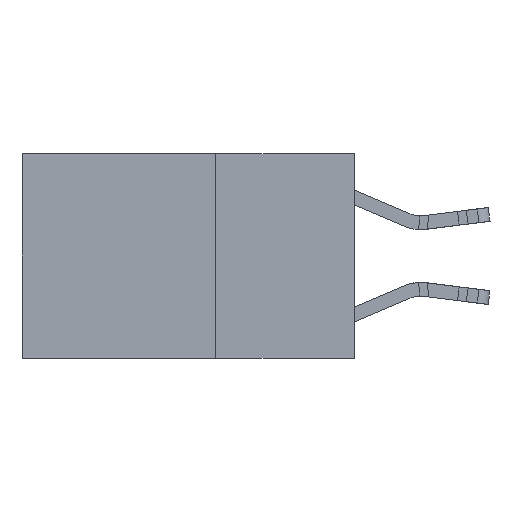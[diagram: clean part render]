
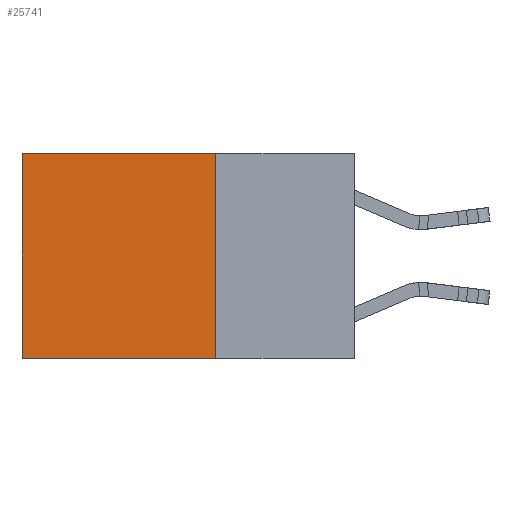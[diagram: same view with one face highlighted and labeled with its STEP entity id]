
A CAD part, left-side view. The second image highlights one B-rep face of the part: STEP entity #25741.
In plain terms, the highlighted planar face has unit normal (-1, 0, 0).
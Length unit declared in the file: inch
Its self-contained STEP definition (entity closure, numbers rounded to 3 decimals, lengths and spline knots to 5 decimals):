
#774 = VECTOR ( 'NONE', #12331, 39.37008 ) ;
#1346 = VERTEX_POINT ( 'NONE', #7805 ) ;
#3901 = LINE ( 'NONE', #20102, #15450 ) ;
#4972 = LINE ( 'NONE', #28841, #12006 ) ;
#5324 = DIRECTION ( 'NONE',  ( 0., 0., -1. ) ) ;
#5791 = ORIENTED_EDGE ( 'NONE', *, *, #26344, .F. ) ;
#7805 = CARTESIAN_POINT ( 'NONE',  ( 0.2625, 0.25, -0.37 ) ) ;
#8162 = VERTEX_POINT ( 'NONE', #11257 ) ;
#8326 = EDGE_CURVE ( 'NONE', #1346, #24345, #26204, .T. ) ;
#10765 = LINE ( 'NONE', #12614, #16415 ) ;
#11257 = CARTESIAN_POINT ( 'NONE',  ( 0.2625, 0.6, 0. ) ) ;
#12006 = VECTOR ( 'NONE', #23373, 39.37008 ) ;
#12331 = DIRECTION ( 'NONE',  ( 0., 1., 0. ) ) ;
#12614 = CARTESIAN_POINT ( 'NONE',  ( 0.2625, 0.25, 0. ) ) ;
#12901 = EDGE_LOOP ( 'NONE', ( #26995, #19051, #5791, #21769 ) ) ;
#13776 = EDGE_CURVE ( 'NONE', #8162, #24345, #4972, .T. ) ;
#14647 = CARTESIAN_POINT ( 'NONE',  ( 0.2625, 0.25, -0.37 ) ) ;
#14826 = DIRECTION ( 'NONE',  ( 1., 0., 0. ) ) ;
#15252 = DIRECTION ( 'NONE',  ( 0., 0., -1. ) ) ;
#15409 = DIRECTION ( 'NONE',  ( 0., 1., 0. ) ) ;
#15450 = VECTOR ( 'NONE', #15409, 39.37008 ) ;
#16415 = VECTOR ( 'NONE', #15252, 39.37008 ) ;
#16723 = FACE_OUTER_BOUND ( 'NONE', #12901, .T. ) ;
#17177 = PLANE ( 'NONE',  #27354 ) ;
#19051 = ORIENTED_EDGE ( 'NONE', *, *, #8326, .F. ) ;
#20066 = VERTEX_POINT ( 'NONE', #28333 ) ;
#20102 = CARTESIAN_POINT ( 'NONE',  ( 0.2625, 0.25, 0. ) ) ;
#21769 = ORIENTED_EDGE ( 'NONE', *, *, #27733, .T. ) ;
#21981 = CARTESIAN_POINT ( 'NONE',  ( 0.2625, 0.6, -0.37 ) ) ;
#23373 = DIRECTION ( 'NONE',  ( 0., 0., -1. ) ) ;
#24345 = VERTEX_POINT ( 'NONE', #21981 ) ;
#25741 = ADVANCED_FACE ( 'NONE', ( #16723 ), #17177, .F. ) ;
#26204 = LINE ( 'NONE', #14647, #774 ) ;
#26344 = EDGE_CURVE ( 'NONE', #20066, #1346, #10765, .T. ) ;
#26845 = CARTESIAN_POINT ( 'NONE',  ( 0.2625, 0.25, 0. ) ) ;
#26995 = ORIENTED_EDGE ( 'NONE', *, *, #13776, .T. ) ;
#27354 = AXIS2_PLACEMENT_3D ( 'NONE', #26845, #14826, #5324 ) ;
#27733 = EDGE_CURVE ( 'NONE', #20066, #8162, #3901, .T. ) ;
#28333 = CARTESIAN_POINT ( 'NONE',  ( 0.2625, 0.25, 0. ) ) ;
#28841 = CARTESIAN_POINT ( 'NONE',  ( 0.2625, 0.6, 0. ) ) ;
